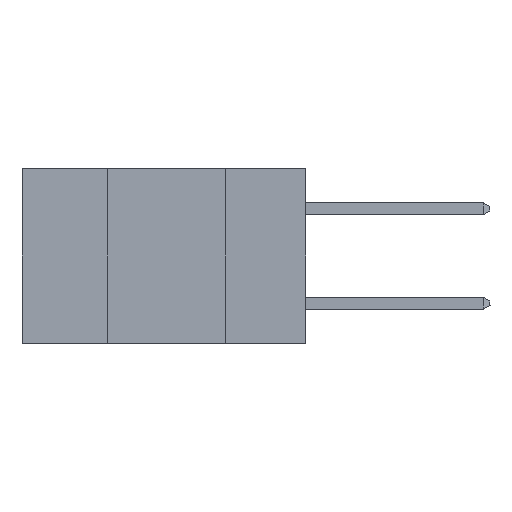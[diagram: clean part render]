
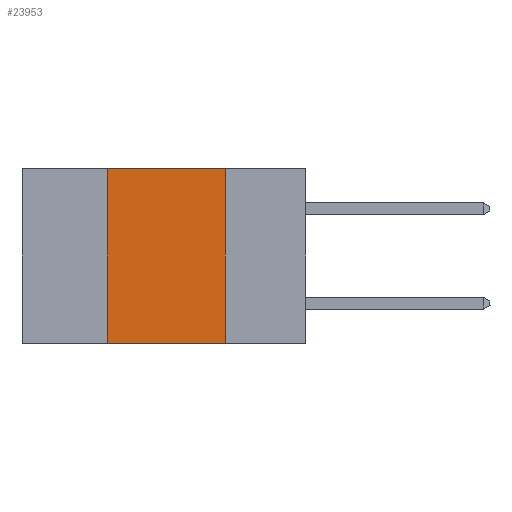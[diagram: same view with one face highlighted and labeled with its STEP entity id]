
A CAD part, left-side view. The second image highlights one B-rep face of the part: STEP entity #23953.
In plain terms, the highlighted planar face has unit normal (-1, 0, 0).
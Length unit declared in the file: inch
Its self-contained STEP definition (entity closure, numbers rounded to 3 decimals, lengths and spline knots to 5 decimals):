
#618 = CARTESIAN_POINT ( 'NONE',  ( 0., 0.17, 0. ) ) ;
#826 = EDGE_LOOP ( 'NONE', ( #8833, #9900, #12354, #1286 ) ) ;
#1286 = ORIENTED_EDGE ( 'NONE', *, *, #10935, .T. ) ;
#1385 = PLANE ( 'NONE',  #3687 ) ;
#1463 = DIRECTION ( 'NONE',  ( 0., -1., 0. ) ) ;
#3392 = DIRECTION ( 'NONE',  ( 1., 0., 0. ) ) ;
#3687 = AXIS2_PLACEMENT_3D ( 'NONE', #15021, #3392, #16955 ) ;
#4492 = VECTOR ( 'NONE', #11474, 39.37008 ) ;
#7108 = CARTESIAN_POINT ( 'NONE',  ( 0., 0.42, 0. ) ) ;
#8087 = VECTOR ( 'NONE', #23752, 39.37008 ) ;
#8777 = DIRECTION ( 'NONE',  ( 0., -1., 0. ) ) ;
#8833 = ORIENTED_EDGE ( 'NONE', *, *, #19178, .F. ) ;
#9375 = CARTESIAN_POINT ( 'NONE',  ( 0., 0.17, 0. ) ) ;
#9900 = ORIENTED_EDGE ( 'NONE', *, *, #16977, .F. ) ;
#10050 = FACE_OUTER_BOUND ( 'NONE', #826, .T. ) ;
#10074 = CARTESIAN_POINT ( 'NONE',  ( 0., 0.42, -0.37 ) ) ;
#10935 = EDGE_CURVE ( 'NONE', #16718, #12181, #18731, .T. ) ;
#11474 = DIRECTION ( 'NONE',  ( 0., 0., 1. ) ) ;
#12181 = VERTEX_POINT ( 'NONE', #22854 ) ;
#12201 = EDGE_CURVE ( 'NONE', #16718, #23856, #14794, .T. ) ;
#12354 = ORIENTED_EDGE ( 'NONE', *, *, #12201, .F. ) ;
#13153 = LINE ( 'NONE', #618, #8087 ) ;
#13933 = VECTOR ( 'NONE', #1463, 39.37008 ) ;
#14794 = LINE ( 'NONE', #20930, #4492 ) ;
#15021 = CARTESIAN_POINT ( 'NONE',  ( 0., 0.6, 0. ) ) ;
#15092 = CARTESIAN_POINT ( 'NONE',  ( 0., 0.6, -0.37 ) ) ;
#16260 = LINE ( 'NONE', #20177, #16863 ) ;
#16718 = VERTEX_POINT ( 'NONE', #10074 ) ;
#16863 = VECTOR ( 'NONE', #8777, 39.37008 ) ;
#16955 = DIRECTION ( 'NONE',  ( 0., 0., -1. ) ) ;
#16977 = EDGE_CURVE ( 'NONE', #23856, #23153, #16260, .T. ) ;
#18731 = LINE ( 'NONE', #15092, #13933 ) ;
#19178 = EDGE_CURVE ( 'NONE', #23153, #12181, #13153, .T. ) ;
#20177 = CARTESIAN_POINT ( 'NONE',  ( 0., 0.6, 0. ) ) ;
#20930 = CARTESIAN_POINT ( 'NONE',  ( 0., 0.42, 0. ) ) ;
#22854 = CARTESIAN_POINT ( 'NONE',  ( 0., 0.17, -0.37 ) ) ;
#23153 = VERTEX_POINT ( 'NONE', #9375 ) ;
#23752 = DIRECTION ( 'NONE',  ( 0., 0., -1. ) ) ;
#23856 = VERTEX_POINT ( 'NONE', #7108 ) ;
#23953 = ADVANCED_FACE ( 'NONE', ( #10050 ), #1385, .F. ) ;
